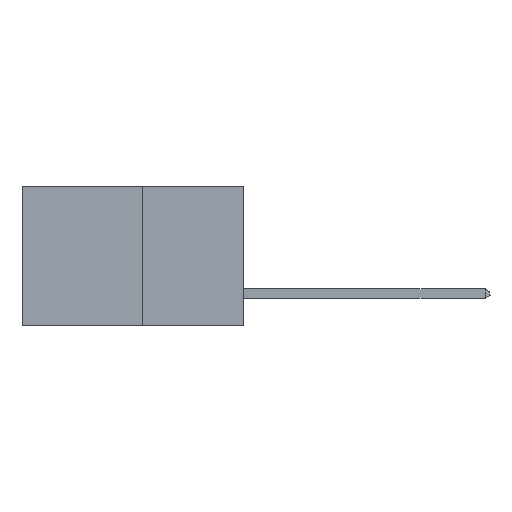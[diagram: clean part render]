
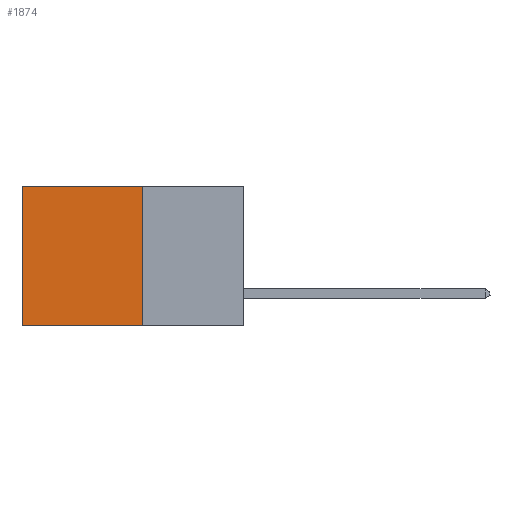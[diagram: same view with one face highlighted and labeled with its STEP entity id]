
A CAD part, left-side view. The second image highlights one B-rep face of the part: STEP entity #1874.
In plain terms, the highlighted planar face has unit normal (-1, 0, 0).
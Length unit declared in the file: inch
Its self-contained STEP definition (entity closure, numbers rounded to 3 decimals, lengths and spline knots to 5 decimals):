
#13 = LINE ( 'NONE', #7314, #8142 ) ;
#132 = CARTESIAN_POINT ( 'NONE',  ( 0.277, 0.59, 0. ) ) ;
#537 = AXIS2_PLACEMENT_3D ( 'NONE', #10810, #11662, #894 ) ;
#894 = DIRECTION ( 'NONE',  ( 0., 0., -1. ) ) ;
#1197 = ORIENTED_EDGE ( 'NONE', *, *, #3685, .F. ) ;
#1261 = EDGE_LOOP ( 'NONE', ( #8487, #13417, #1197, #1917 ) ) ;
#1517 = VERTEX_POINT ( 'NONE', #132 ) ;
#1874 = ADVANCED_FACE ( 'NONE', ( #5245 ), #11725, .F. ) ;
#1917 = ORIENTED_EDGE ( 'NONE', *, *, #10361, .T. ) ;
#2166 = EDGE_CURVE ( 'NONE', #2830, #11895, #6959, .T. ) ;
#2774 = LINE ( 'NONE', #6888, #13856 ) ;
#2830 = VERTEX_POINT ( 'NONE', #11712 ) ;
#3685 = EDGE_CURVE ( 'NONE', #9214, #2830, #13, .T. ) ;
#4060 = VECTOR ( 'NONE', #8208, 39.37008 ) ;
#4065 = CARTESIAN_POINT ( 'NONE',  ( 0.277, 0.27, 0. ) ) ;
#4103 = VECTOR ( 'NONE', #7989, 39.37008 ) ;
#4437 = LINE ( 'NONE', #11151, #4103 ) ;
#5245 = FACE_OUTER_BOUND ( 'NONE', #1261, .T. ) ;
#6888 = CARTESIAN_POINT ( 'NONE',  ( 0.277, 0.27, 0. ) ) ;
#6959 = LINE ( 'NONE', #9930, #4060 ) ;
#7314 = CARTESIAN_POINT ( 'NONE',  ( 0.277, 0.27, -0.37 ) ) ;
#7989 = DIRECTION ( 'NONE',  ( 0., 0., -1. ) ) ;
#8142 = VECTOR ( 'NONE', #9379, 39.37008 ) ;
#8208 = DIRECTION ( 'NONE',  ( 0., 1., 0. ) ) ;
#8487 = ORIENTED_EDGE ( 'NONE', *, *, #13904, .T. ) ;
#9214 = VERTEX_POINT ( 'NONE', #4065 ) ;
#9379 = DIRECTION ( 'NONE',  ( 0., 0., -1. ) ) ;
#9930 = CARTESIAN_POINT ( 'NONE',  ( 0.277, 0.27, -0.37 ) ) ;
#10361 = EDGE_CURVE ( 'NONE', #9214, #1517, #2774, .T. ) ;
#10810 = CARTESIAN_POINT ( 'NONE',  ( 0.277, 0.27, -0.37 ) ) ;
#11151 = CARTESIAN_POINT ( 'NONE',  ( 0.277, 0.59, -0.37 ) ) ;
#11662 = DIRECTION ( 'NONE',  ( 1., 0., 0. ) ) ;
#11712 = CARTESIAN_POINT ( 'NONE',  ( 0.277, 0.27, -0.37 ) ) ;
#11725 = PLANE ( 'NONE',  #537 ) ;
#11895 = VERTEX_POINT ( 'NONE', #13020 ) ;
#13020 = CARTESIAN_POINT ( 'NONE',  ( 0.277, 0.59, -0.37 ) ) ;
#13277 = DIRECTION ( 'NONE',  ( 0., 1., 0. ) ) ;
#13417 = ORIENTED_EDGE ( 'NONE', *, *, #2166, .F. ) ;
#13856 = VECTOR ( 'NONE', #13277, 39.37008 ) ;
#13904 = EDGE_CURVE ( 'NONE', #1517, #11895, #4437, .T. ) ;
